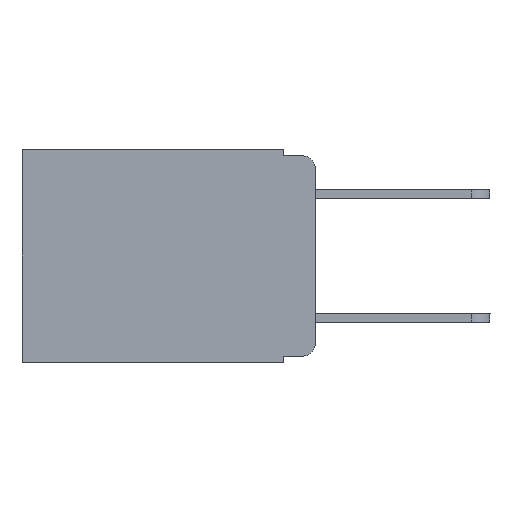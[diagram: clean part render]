
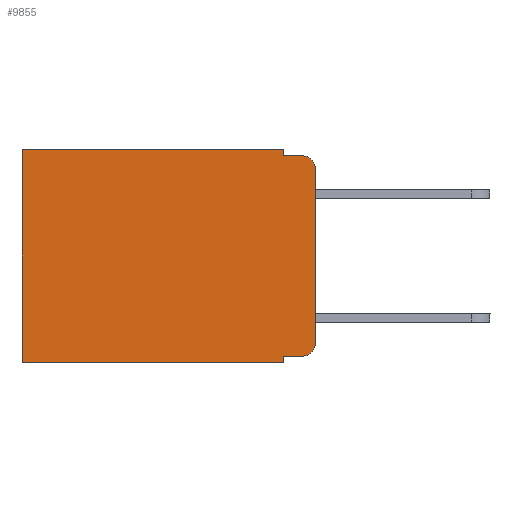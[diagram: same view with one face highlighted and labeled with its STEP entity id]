
A CAD part, left-side view. The second image highlights one B-rep face of the part: STEP entity #9855.
In plain terms, the highlighted planar face has unit normal (-1, 0, 0).
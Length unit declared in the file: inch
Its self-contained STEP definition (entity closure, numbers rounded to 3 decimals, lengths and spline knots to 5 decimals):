
#1760 = VERTEX_POINT ( 'NONE', #10091 ) ;
#1773 = VECTOR ( 'NONE', #9895, 39.37008 ) ;
#2008 = VECTOR ( 'NONE', #4366, 39.37008 ) ;
#2023 = CARTESIAN_POINT ( 'NONE',  ( 0.298, 0.473, 0. ) ) ;
#2312 = VERTEX_POINT ( 'NONE', #2023 ) ;
#2323 = CARTESIAN_POINT ( 'NONE',  ( 0.298, 0.02, -0.333 ) ) ;
#2558 = VECTOR ( 'NONE', #10405, 39.37008 ) ;
#2580 = AXIS2_PLACEMENT_3D ( 'NONE', #3450, #3514, #17732 ) ;
#2692 = CARTESIAN_POINT ( 'NONE',  ( 0.298, 0.051, -0.333 ) ) ;
#3010 = VERTEX_POINT ( 'NONE', #2323 ) ;
#3143 = LINE ( 'NONE', #10111, #14025 ) ;
#3450 = CARTESIAN_POINT ( 'NONE',  ( 0.298, 0.02, -0.313 ) ) ;
#3463 = CARTESIAN_POINT ( 'NONE',  ( 0.298, 0.051, 0. ) ) ;
#3514 = DIRECTION ( 'NONE',  ( -1., 0., 0. ) ) ;
#3724 = EDGE_CURVE ( 'NONE', #1760, #15539, #3143, .T. ) ;
#3904 = VERTEX_POINT ( 'NONE', #11748 ) ;
#3980 = LINE ( 'NONE', #8283, #6919 ) ;
#4155 = DIRECTION ( 'NONE',  ( 0., -1., 0. ) ) ;
#4250 = CARTESIAN_POINT ( 'NONE',  ( 0.298, 0.473, 0. ) ) ;
#4366 = DIRECTION ( 'NONE',  ( 0., 0., -1. ) ) ;
#4371 = FACE_OUTER_BOUND ( 'NONE', #12274, .T. ) ;
#4476 = LINE ( 'NONE', #2692, #11266 ) ;
#4683 = ORIENTED_EDGE ( 'NONE', *, *, #12137, .F. ) ;
#4975 = DIRECTION ( 'NONE',  ( 0., 0., -1. ) ) ;
#5062 = EDGE_CURVE ( 'NONE', #16745, #3904, #12432, .T. ) ;
#5430 = ORIENTED_EDGE ( 'NONE', *, *, #6201, .T. ) ;
#5591 = LINE ( 'NONE', #8446, #1773 ) ;
#5826 = LINE ( 'NONE', #4250, #2008 ) ;
#5944 = VERTEX_POINT ( 'NONE', #12536 ) ;
#6201 = EDGE_CURVE ( 'NONE', #13052, #3010, #4476, .T. ) ;
#6206 = ORIENTED_EDGE ( 'NONE', *, *, #9976, .F. ) ;
#6612 = CARTESIAN_POINT ( 'NONE',  ( 0.298, 0.051, -0.333 ) ) ;
#6763 = EDGE_CURVE ( 'NONE', #1760, #13691, #17563, .T. ) ;
#6893 = CARTESIAN_POINT ( 'NONE',  ( 0.298, 0.02, -0.01 ) ) ;
#6919 = VECTOR ( 'NONE', #9805, 39.37008 ) ;
#7228 = CARTESIAN_POINT ( 'NONE',  ( 0.298, 0., 0. ) ) ;
#8214 = EDGE_CURVE ( 'NONE', #16745, #2312, #3980, .T. ) ;
#8217 = ORIENTED_EDGE ( 'NONE', *, *, #3724, .F. ) ;
#8283 = CARTESIAN_POINT ( 'NONE',  ( 0.298, 0., 0. ) ) ;
#8446 = CARTESIAN_POINT ( 'NONE',  ( 0.298, 0., -0.343 ) ) ;
#8494 = ORIENTED_EDGE ( 'NONE', *, *, #5062, .F. ) ;
#8687 = DIRECTION ( 'NONE',  ( 0., 0., -1. ) ) ;
#8952 = CARTESIAN_POINT ( 'NONE',  ( 0.298, 0.051, 0. ) ) ;
#9286 = VERTEX_POINT ( 'NONE', #12943 ) ;
#9731 = AXIS2_PLACEMENT_3D ( 'NONE', #7228, #17346, #8687 ) ;
#9805 = DIRECTION ( 'NONE',  ( 0., 1., 0. ) ) ;
#9855 = ADVANCED_FACE ( 'NONE', ( #4371 ), #17218, .F. ) ;
#9895 = DIRECTION ( 'NONE',  ( 0., 1., 0. ) ) ;
#9918 = CARTESIAN_POINT ( 'NONE',  ( 0.298, 0.02, -0.03 ) ) ;
#9976 = EDGE_CURVE ( 'NONE', #13052, #9286, #13632, .T. ) ;
#9997 = LINE ( 'NONE', #15684, #18328 ) ;
#10091 = CARTESIAN_POINT ( 'NONE',  ( 0.298, 0., -0.03 ) ) ;
#10111 = CARTESIAN_POINT ( 'NONE',  ( 0.298, 0., 0. ) ) ;
#10405 = DIRECTION ( 'NONE',  ( 0., 0., -1. ) ) ;
#11266 = VECTOR ( 'NONE', #12980, 39.37008 ) ;
#11378 = DIRECTION ( 'NONE',  ( -1., 0., 0. ) ) ;
#11748 = CARTESIAN_POINT ( 'NONE',  ( 0.298, 0.051, -0.01 ) ) ;
#11980 = AXIS2_PLACEMENT_3D ( 'NONE', #9918, #11378, #12838 ) ;
#12137 = EDGE_CURVE ( 'NONE', #3904, #13691, #9997, .T. ) ;
#12274 = EDGE_LOOP ( 'NONE', ( #8217, #14567, #4683, #8494, #13285, #18562, #15809, #6206, #5430, #15249 ) ) ;
#12432 = LINE ( 'NONE', #3463, #18082 ) ;
#12536 = CARTESIAN_POINT ( 'NONE',  ( 0.298, 0.473, -0.343 ) ) ;
#12708 = CARTESIAN_POINT ( 'NONE',  ( 0.298, 0., -0.313 ) ) ;
#12838 = DIRECTION ( 'NONE',  ( 0., 0., -1. ) ) ;
#12943 = CARTESIAN_POINT ( 'NONE',  ( 0.298, 0.051, -0.343 ) ) ;
#12980 = DIRECTION ( 'NONE',  ( 0., -1., 0. ) ) ;
#13052 = VERTEX_POINT ( 'NONE', #6612 ) ;
#13285 = ORIENTED_EDGE ( 'NONE', *, *, #8214, .T. ) ;
#13632 = LINE ( 'NONE', #8952, #2558 ) ;
#13691 = VERTEX_POINT ( 'NONE', #6893 ) ;
#14025 = VECTOR ( 'NONE', #17256, 39.37008 ) ;
#14334 = EDGE_CURVE ( 'NONE', #9286, #5944, #5591, .T. ) ;
#14567 = ORIENTED_EDGE ( 'NONE', *, *, #6763, .T. ) ;
#14646 = CARTESIAN_POINT ( 'NONE',  ( 0.298, 0.051, 0. ) ) ;
#14794 = CIRCLE ( 'NONE', #2580, 0.02 ) ;
#15028 = EDGE_CURVE ( 'NONE', #2312, #5944, #5826, .T. ) ;
#15249 = ORIENTED_EDGE ( 'NONE', *, *, #17497, .T. ) ;
#15539 = VERTEX_POINT ( 'NONE', #12708 ) ;
#15684 = CARTESIAN_POINT ( 'NONE',  ( 0.298, 0.051, -0.01 ) ) ;
#15809 = ORIENTED_EDGE ( 'NONE', *, *, #14334, .F. ) ;
#16745 = VERTEX_POINT ( 'NONE', #14646 ) ;
#17218 = PLANE ( 'NONE',  #9731 ) ;
#17256 = DIRECTION ( 'NONE',  ( 0., 0., -1. ) ) ;
#17346 = DIRECTION ( 'NONE',  ( 1., 0., 0. ) ) ;
#17497 = EDGE_CURVE ( 'NONE', #3010, #15539, #14794, .T. ) ;
#17563 = CIRCLE ( 'NONE', #11980, 0.02 ) ;
#17732 = DIRECTION ( 'NONE',  ( 0., 0., -1. ) ) ;
#18082 = VECTOR ( 'NONE', #4975, 39.37008 ) ;
#18328 = VECTOR ( 'NONE', #4155, 39.37008 ) ;
#18562 = ORIENTED_EDGE ( 'NONE', *, *, #15028, .T. ) ;
